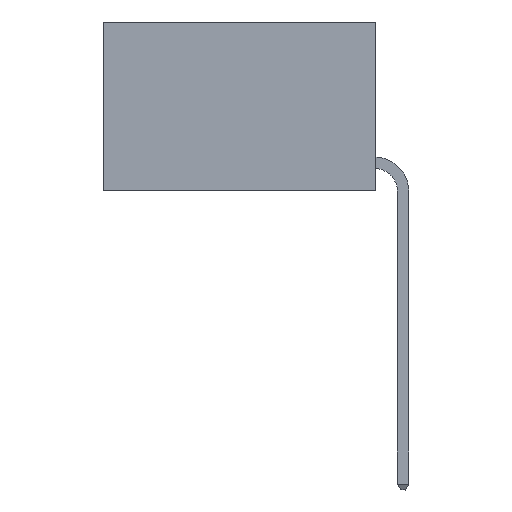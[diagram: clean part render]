
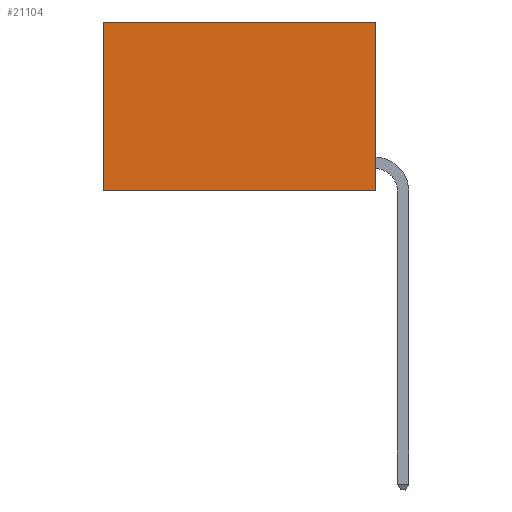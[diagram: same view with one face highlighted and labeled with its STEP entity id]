
A CAD part, left-side view. The second image highlights one B-rep face of the part: STEP entity #21104.
In plain terms, the highlighted planar face has unit normal (-1, 0, 0).
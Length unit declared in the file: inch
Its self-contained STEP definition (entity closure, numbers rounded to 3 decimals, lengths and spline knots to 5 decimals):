
#515 = LINE ( 'NONE', #23233, #21993 ) ;
#1393 = LINE ( 'NONE', #13181, #16770 ) ;
#1574 = EDGE_CURVE ( 'NONE', #22993, #19175, #24049, .T. ) ;
#2286 = PLANE ( 'NONE',  #25478 ) ;
#2381 = EDGE_LOOP ( 'NONE', ( #9510, #22736, #5867, #24707 ) ) ;
#4390 = DIRECTION ( 'NONE',  ( 1., 0., 0. ) ) ;
#5867 = ORIENTED_EDGE ( 'NONE', *, *, #12730, .F. ) ;
#6942 = VECTOR ( 'NONE', #25550, 39.37008 ) ;
#7454 = FACE_OUTER_BOUND ( 'NONE', #2381, .T. ) ;
#9510 = ORIENTED_EDGE ( 'NONE', *, *, #1574, .T. ) ;
#10632 = CARTESIAN_POINT ( 'NONE',  ( 0.2625, 0., 0. ) ) ;
#12502 = VERTEX_POINT ( 'NONE', #22191 ) ;
#12730 = EDGE_CURVE ( 'NONE', #12502, #19646, #21806, .T. ) ;
#12987 = DIRECTION ( 'NONE',  ( 0., 1., 0. ) ) ;
#13181 = CARTESIAN_POINT ( 'NONE',  ( 0.2625, 0., 0. ) ) ;
#16428 = CARTESIAN_POINT ( 'NONE',  ( 0.2625, 0.6, 0. ) ) ;
#16727 = CARTESIAN_POINT ( 'NONE',  ( 0.2625, 0.6, -0.37 ) ) ;
#16770 = VECTOR ( 'NONE', #25492, 39.37008 ) ;
#18964 = DIRECTION ( 'NONE',  ( 0., 0., -1. ) ) ;
#19175 = VERTEX_POINT ( 'NONE', #16727 ) ;
#19646 = VERTEX_POINT ( 'NONE', #22228 ) ;
#20838 = CARTESIAN_POINT ( 'NONE',  ( 0.2625, 0., 0. ) ) ;
#21104 = ADVANCED_FACE ( 'NONE', ( #7454 ), #2286, .F. ) ;
#21169 = EDGE_CURVE ( 'NONE', #19646, #19175, #515, .T. ) ;
#21806 = LINE ( 'NONE', #20838, #26567 ) ;
#21993 = VECTOR ( 'NONE', #12987, 39.37008 ) ;
#22191 = CARTESIAN_POINT ( 'NONE',  ( 0.2625, 0., 0. ) ) ;
#22228 = CARTESIAN_POINT ( 'NONE',  ( 0.2625, 0., -0.37 ) ) ;
#22736 = ORIENTED_EDGE ( 'NONE', *, *, #21169, .F. ) ;
#22808 = DIRECTION ( 'NONE',  ( 0., 0., -1. ) ) ;
#22993 = VERTEX_POINT ( 'NONE', #25974 ) ;
#23233 = CARTESIAN_POINT ( 'NONE',  ( 0.2625, 0., -0.37 ) ) ;
#23508 = EDGE_CURVE ( 'NONE', #12502, #22993, #1393, .T. ) ;
#24049 = LINE ( 'NONE', #16428, #6942 ) ;
#24707 = ORIENTED_EDGE ( 'NONE', *, *, #23508, .T. ) ;
#25478 = AXIS2_PLACEMENT_3D ( 'NONE', #10632, #4390, #18964 ) ;
#25492 = DIRECTION ( 'NONE',  ( 0., 1., 0. ) ) ;
#25550 = DIRECTION ( 'NONE',  ( 0., 0., -1. ) ) ;
#25974 = CARTESIAN_POINT ( 'NONE',  ( 0.2625, 0.6, 0. ) ) ;
#26567 = VECTOR ( 'NONE', #22808, 39.37008 ) ;
